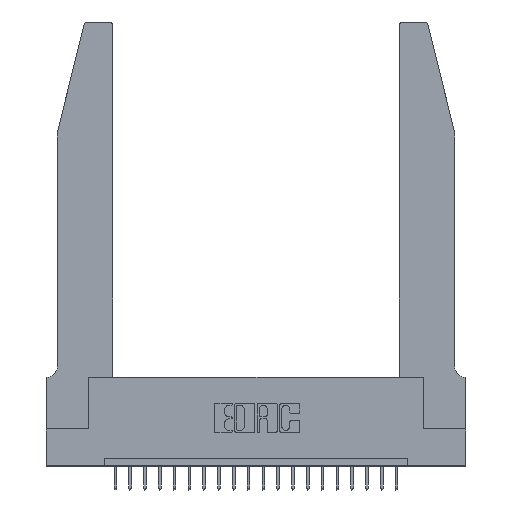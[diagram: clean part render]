
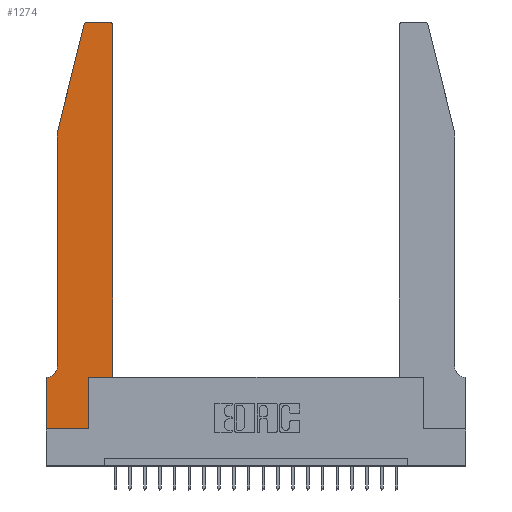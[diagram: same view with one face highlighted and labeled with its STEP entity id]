
A CAD part, top view. The second image highlights one B-rep face of the part: STEP entity #1274.
In plain terms, the highlighted planar face has unit normal (0, 0, 1).
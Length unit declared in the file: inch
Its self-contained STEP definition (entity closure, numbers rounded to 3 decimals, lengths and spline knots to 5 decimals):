
#95 = CARTESIAN_POINT ( 'NONE',  ( 0.284, 2.72, 0.37 ) ) ;
#144 = CARTESIAN_POINT ( 'NONE',  ( 0.2865, 0.35, 0.37 ) ) ;
#168 = LINE ( 'NONE', #20606, #22525 ) ;
#329 = ORIENTED_EDGE ( 'NONE', *, *, #10408, .T. ) ;
#737 = CARTESIAN_POINT ( 'NONE',  ( 0.0055, 0.42, 0.37 ) ) ;
#1166 = LINE ( 'NONE', #9812, #2001 ) ;
#1169 = DIRECTION ( 'NONE',  ( 1., 0., 0. ) ) ;
#1178 = DIRECTION ( 'NONE',  ( -1., 0., 0. ) ) ;
#1274 = ADVANCED_FACE ( 'NONE', ( #3468 ), #18176, .T. ) ;
#1317 = EDGE_CURVE ( 'NONE', #17714, #19568, #7119, .T. ) ;
#1979 = CARTESIAN_POINT ( 'NONE',  ( 0.0755, 0.42, 0.37 ) ) ;
#2001 = VECTOR ( 'NONE', #18349, 39.37008 ) ;
#2324 = EDGE_CURVE ( 'NONE', #21295, #16634, #14175, .T. ) ;
#3073 = CARTESIAN_POINT ( 'NONE',  ( 0.4505, 2.72, 0.37 ) ) ;
#3257 = ORIENTED_EDGE ( 'NONE', *, *, #15543, .T. ) ;
#3287 = CARTESIAN_POINT ( 'NONE',  ( 0.2865, 0.35, 0.37 ) ) ;
#3347 = VERTEX_POINT ( 'NONE', #5977 ) ;
#3468 = FACE_OUTER_BOUND ( 'NONE', #7977, .T. ) ;
#3689 = DIRECTION ( 'NONE',  ( 1., 0., 0. ) ) ;
#3735 = CIRCLE ( 'NONE', #5416, 0.03 ) ;
#4106 = DIRECTION ( 'NONE',  ( 0., 0., 1. ) ) ;
#4165 = CARTESIAN_POINT ( 'NONE',  ( 0., 0., 0.37 ) ) ;
#4175 = DIRECTION ( 'NONE',  ( -1., 0., 0. ) ) ;
#5416 = AXIS2_PLACEMENT_3D ( 'NONE', #20520, #11785, #1169 ) ;
#5888 = ORIENTED_EDGE ( 'NONE', *, *, #12567, .T. ) ;
#5973 = CARTESIAN_POINT ( 'NONE',  ( 0.284, 2.75, 0.37 ) ) ;
#5977 = CARTESIAN_POINT ( 'NONE',  ( 0.25487, 2.72718, 0.37 ) ) ;
#6146 = CARTESIAN_POINT ( 'NONE',  ( 0., 0.35, 0.37 ) ) ;
#6533 = EDGE_CURVE ( 'NONE', #21183, #17352, #17217, .T. ) ;
#6635 = CARTESIAN_POINT ( 'NONE',  ( 0.4505, 0.35, 0.37 ) ) ;
#6893 = VERTEX_POINT ( 'NONE', #14971 ) ;
#7059 = LINE ( 'NONE', #144, #20182 ) ;
#7119 = CIRCLE ( 'NONE', #20313, 0.07 ) ;
#7165 = EDGE_CURVE ( 'NONE', #19568, #6893, #11406, .T. ) ;
#7292 = CARTESIAN_POINT ( 'NONE',  ( 0.4505, 0.35, 0.37 ) ) ;
#7622 = ORIENTED_EDGE ( 'NONE', *, *, #9416, .T. ) ;
#7808 = DIRECTION ( 'NONE',  ( 0., 1., 0. ) ) ;
#7977 = EDGE_LOOP ( 'NONE', ( #5888, #329, #3257, #7622, #8831, #9402, #17953, #12791, #15875, #22337, #12959, #12168 ) ) ;
#8238 = DIRECTION ( 'NONE',  ( 0., -1., 0. ) ) ;
#8831 = ORIENTED_EDGE ( 'NONE', *, *, #1317, .T. ) ;
#8969 = VERTEX_POINT ( 'NONE', #19232 ) ;
#9402 = ORIENTED_EDGE ( 'NONE', *, *, #7165, .T. ) ;
#9416 = EDGE_CURVE ( 'NONE', #8969, #17714, #19536, .T. ) ;
#9790 = AXIS2_PLACEMENT_3D ( 'NONE', #6146, #4106, #12945 ) ;
#9812 = CARTESIAN_POINT ( 'NONE',  ( 0.0755, 2., 0.37 ) ) ;
#9961 = CARTESIAN_POINT ( 'NONE',  ( 0.0755, 0.35, 0.37 ) ) ;
#10408 = EDGE_CURVE ( 'NONE', #20800, #3347, #19317, .T. ) ;
#11361 = LINE ( 'NONE', #7292, #22352 ) ;
#11406 = LINE ( 'NONE', #9961, #15538 ) ;
#11785 = DIRECTION ( 'NONE',  ( 0., 0., 1. ) ) ;
#12168 = ORIENTED_EDGE ( 'NONE', *, *, #14555, .T. ) ;
#12309 = DIRECTION ( 'NONE',  ( 0., -1., 0. ) ) ;
#12475 = DIRECTION ( 'NONE',  ( 0., 0., 1. ) ) ;
#12567 = EDGE_CURVE ( 'NONE', #16007, #20800, #168, .T. ) ;
#12791 = ORIENTED_EDGE ( 'NONE', *, *, #2324, .T. ) ;
#12945 = DIRECTION ( 'NONE',  ( 1., 0., 0. ) ) ;
#12959 = ORIENTED_EDGE ( 'NONE', *, *, #6533, .T. ) ;
#13169 = VECTOR ( 'NONE', #8238, 39.37008 ) ;
#14175 = LINE ( 'NONE', #19839, #14729 ) ;
#14555 = EDGE_CURVE ( 'NONE', #17352, #16007, #3735, .T. ) ;
#14637 = DIRECTION ( 'NONE',  ( 1., 0., 0. ) ) ;
#14729 = VECTOR ( 'NONE', #14637, 39.37008 ) ;
#14897 = DIRECTION ( 'NONE',  ( 0., 1., 0. ) ) ;
#14971 = CARTESIAN_POINT ( 'NONE',  ( 0., 0.35, 0.37 ) ) ;
#15537 = CARTESIAN_POINT ( 'NONE',  ( 0.0055, 0.35, 0.37 ) ) ;
#15538 = VECTOR ( 'NONE', #18193, 39.37008 ) ;
#15543 = EDGE_CURVE ( 'NONE', #3347, #8969, #1166, .T. ) ;
#15809 = AXIS2_PLACEMENT_3D ( 'NONE', #95, #12475, #17837 ) ;
#15875 = ORIENTED_EDGE ( 'NONE', *, *, #20563, .T. ) ;
#16007 = VERTEX_POINT ( 'NONE', #21485 ) ;
#16113 = CARTESIAN_POINT ( 'NONE',  ( 0.4505, 0.35, 0.37 ) ) ;
#16587 = VERTEX_POINT ( 'NONE', #3287 ) ;
#16634 = VERTEX_POINT ( 'NONE', #20766 ) ;
#16655 = VECTOR ( 'NONE', #7808, 39.37008 ) ;
#17217 = LINE ( 'NONE', #6635, #16655 ) ;
#17246 = EDGE_CURVE ( 'NONE', #6893, #21295, #17847, .T. ) ;
#17352 = VERTEX_POINT ( 'NONE', #3073 ) ;
#17714 = VERTEX_POINT ( 'NONE', #1979 ) ;
#17837 = DIRECTION ( 'NONE',  ( 1., 0., 0. ) ) ;
#17847 = LINE ( 'NONE', #4165, #13169 ) ;
#17901 = VECTOR ( 'NONE', #12309, 39.37008 ) ;
#17953 = ORIENTED_EDGE ( 'NONE', *, *, #17246, .T. ) ;
#18176 = PLANE ( 'NONE',  #9790 ) ;
#18193 = DIRECTION ( 'NONE',  ( -1., 0., 0. ) ) ;
#18349 = DIRECTION ( 'NONE',  ( -0.239, -0.971, 0. ) ) ;
#19232 = CARTESIAN_POINT ( 'NONE',  ( 0.0755, 2., 0.37 ) ) ;
#19317 = CIRCLE ( 'NONE', #15809, 0.03 ) ;
#19422 = CARTESIAN_POINT ( 'NONE',  ( 0.0755, 2., 0.37 ) ) ;
#19536 = LINE ( 'NONE', #19422, #17901 ) ;
#19568 = VERTEX_POINT ( 'NONE', #15537 ) ;
#19839 = CARTESIAN_POINT ( 'NONE',  ( 0., 0., 0.37 ) ) ;
#19938 = DIRECTION ( 'NONE',  ( 0., 0., -1. ) ) ;
#20148 = CARTESIAN_POINT ( 'NONE',  ( 0., 0., 0.37 ) ) ;
#20182 = VECTOR ( 'NONE', #14897, 39.37008 ) ;
#20313 = AXIS2_PLACEMENT_3D ( 'NONE', #737, #19938, #4175 ) ;
#20520 = CARTESIAN_POINT ( 'NONE',  ( 0.4205, 2.72, 0.37 ) ) ;
#20563 = EDGE_CURVE ( 'NONE', #16634, #16587, #7059, .T. ) ;
#20606 = CARTESIAN_POINT ( 'NONE',  ( 0.2605, 2.75, 0.37 ) ) ;
#20766 = CARTESIAN_POINT ( 'NONE',  ( 0.2865, 0., 0.37 ) ) ;
#20800 = VERTEX_POINT ( 'NONE', #5973 ) ;
#21183 = VERTEX_POINT ( 'NONE', #16113 ) ;
#21295 = VERTEX_POINT ( 'NONE', #20148 ) ;
#21485 = CARTESIAN_POINT ( 'NONE',  ( 0.4205, 2.75, 0.37 ) ) ;
#21616 = EDGE_CURVE ( 'NONE', #16587, #21183, #11361, .T. ) ;
#22337 = ORIENTED_EDGE ( 'NONE', *, *, #21616, .T. ) ;
#22352 = VECTOR ( 'NONE', #3689, 39.37008 ) ;
#22525 = VECTOR ( 'NONE', #1178, 39.37008 ) ;
